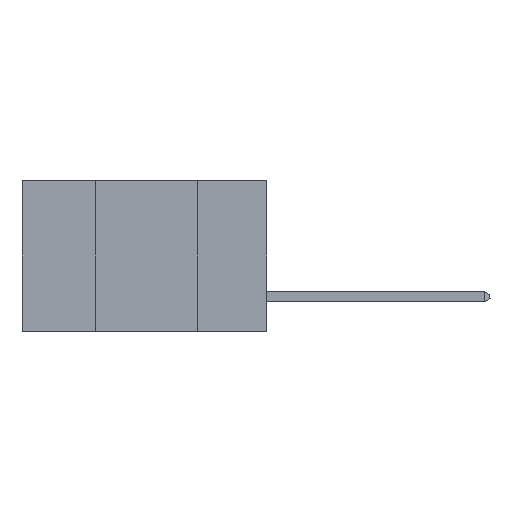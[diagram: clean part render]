
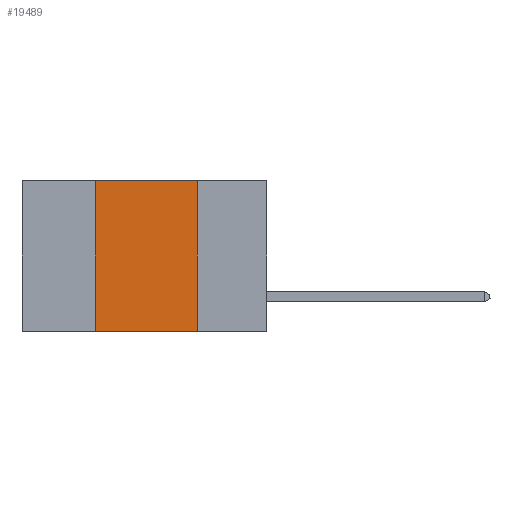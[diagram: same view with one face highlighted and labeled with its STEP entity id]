
A CAD part, left-side view. The second image highlights one B-rep face of the part: STEP entity #19489.
In plain terms, the highlighted planar face has unit normal (-1, 0, 0).
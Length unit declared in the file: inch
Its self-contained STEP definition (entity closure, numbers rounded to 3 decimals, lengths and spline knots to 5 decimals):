
#366 = VERTEX_POINT ( 'NONE', #12694 ) ;
#1044 = EDGE_CURVE ( 'NONE', #366, #19507, #9589, .T. ) ;
#1469 = LINE ( 'NONE', #21378, #16000 ) ;
#1837 = DIRECTION ( 'NONE',  ( 0., -1., 0. ) ) ;
#2298 = CARTESIAN_POINT ( 'NONE',  ( 0., 0.42, 0. ) ) ;
#3805 = DIRECTION ( 'NONE',  ( 0., 0., -1. ) ) ;
#4048 = DIRECTION ( 'NONE',  ( 0., 0., 1. ) ) ;
#4503 = AXIS2_PLACEMENT_3D ( 'NONE', #26140, #24117, #11481 ) ;
#5136 = LINE ( 'NONE', #18920, #15765 ) ;
#6263 = ORIENTED_EDGE ( 'NONE', *, *, #8793, .F. ) ;
#6759 = VERTEX_POINT ( 'NONE', #7704 ) ;
#7146 = CARTESIAN_POINT ( 'NONE',  ( 0., 0.17, -0.37 ) ) ;
#7704 = CARTESIAN_POINT ( 'NONE',  ( 0., 0.17, 0. ) ) ;
#7749 = LINE ( 'NONE', #14268, #20416 ) ;
#8785 = DIRECTION ( 'NONE',  ( 0., -1., 0. ) ) ;
#8793 = EDGE_CURVE ( 'NONE', #6759, #20872, #7749, .T. ) ;
#9589 = LINE ( 'NONE', #2298, #21256 ) ;
#11120 = EDGE_LOOP ( 'NONE', ( #6263, #15868, #22936, #22916 ) ) ;
#11481 = DIRECTION ( 'NONE',  ( 0., 0., -1. ) ) ;
#12694 = CARTESIAN_POINT ( 'NONE',  ( 0., 0.42, -0.37 ) ) ;
#12889 = FACE_OUTER_BOUND ( 'NONE', #11120, .T. ) ;
#14268 = CARTESIAN_POINT ( 'NONE',  ( 0., 0.17, 0. ) ) ;
#15765 = VECTOR ( 'NONE', #8785, 39.37008 ) ;
#15868 = ORIENTED_EDGE ( 'NONE', *, *, #23090, .F. ) ;
#16000 = VECTOR ( 'NONE', #1837, 39.37008 ) ;
#17840 = EDGE_CURVE ( 'NONE', #366, #20872, #1469, .T. ) ;
#18920 = CARTESIAN_POINT ( 'NONE',  ( 0., 0.6, 0. ) ) ;
#19489 = ADVANCED_FACE ( 'NONE', ( #12889 ), #24305, .F. ) ;
#19507 = VERTEX_POINT ( 'NONE', #26510 ) ;
#20416 = VECTOR ( 'NONE', #3805, 39.37008 ) ;
#20872 = VERTEX_POINT ( 'NONE', #7146 ) ;
#21256 = VECTOR ( 'NONE', #4048, 39.37008 ) ;
#21378 = CARTESIAN_POINT ( 'NONE',  ( 0., 0.6, -0.37 ) ) ;
#22916 = ORIENTED_EDGE ( 'NONE', *, *, #17840, .T. ) ;
#22936 = ORIENTED_EDGE ( 'NONE', *, *, #1044, .F. ) ;
#23090 = EDGE_CURVE ( 'NONE', #19507, #6759, #5136, .T. ) ;
#24117 = DIRECTION ( 'NONE',  ( 1., 0., 0. ) ) ;
#24305 = PLANE ( 'NONE',  #4503 ) ;
#26140 = CARTESIAN_POINT ( 'NONE',  ( 0., 0.6, 0. ) ) ;
#26510 = CARTESIAN_POINT ( 'NONE',  ( 0., 0.42, 0. ) ) ;
